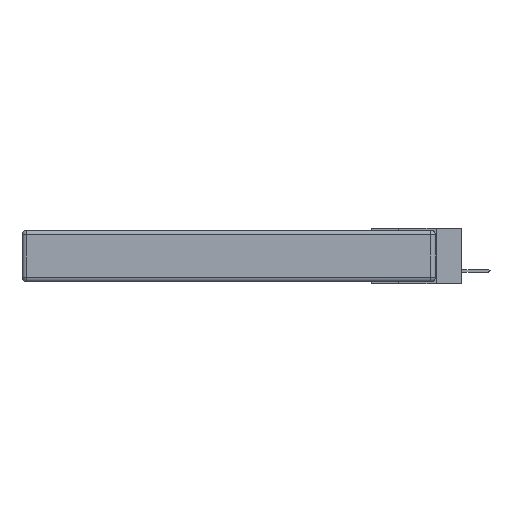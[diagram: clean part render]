
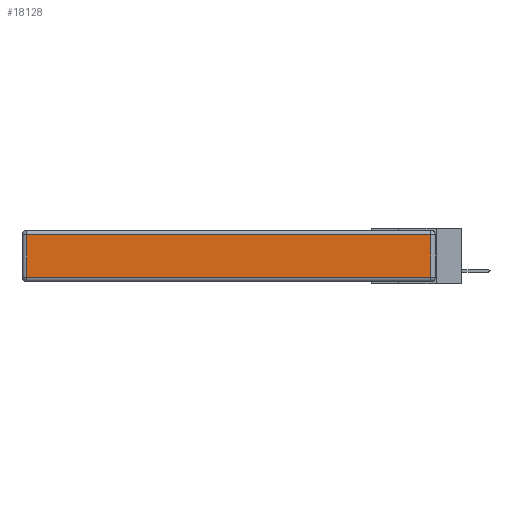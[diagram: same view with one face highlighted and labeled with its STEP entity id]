
A CAD part, left-side view. The second image highlights one B-rep face of the part: STEP entity #18128.
In plain terms, the highlighted planar face has unit normal (-1, 0, 0).
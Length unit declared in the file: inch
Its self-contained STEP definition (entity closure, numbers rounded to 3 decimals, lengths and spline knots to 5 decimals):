
#512 = VERTEX_POINT ( 'NONE', #15172 ) ;
#901 = VERTEX_POINT ( 'NONE', #2842 ) ;
#2226 = FACE_OUTER_BOUND ( 'NONE', #13156, .T. ) ;
#2771 = LINE ( 'NONE', #11736, #21294 ) ;
#2814 = ORIENTED_EDGE ( 'NONE', *, *, #7463, .T. ) ;
#2842 = CARTESIAN_POINT ( 'NONE',  ( 0., 0.03, -0.313 ) ) ;
#4754 = LINE ( 'NONE', #12436, #13782 ) ;
#5283 = DIRECTION ( 'NONE',  ( 0., 1., 0. ) ) ;
#5711 = DIRECTION ( 'NONE',  ( 0., 0., 1. ) ) ;
#6451 = DIRECTION ( 'NONE',  ( 0., 0., -1. ) ) ;
#6588 = ORIENTED_EDGE ( 'NONE', *, *, #10198, .T. ) ;
#7266 = ORIENTED_EDGE ( 'NONE', *, *, #14042, .T. ) ;
#7340 = LINE ( 'NONE', #15498, #22293 ) ;
#7463 = EDGE_CURVE ( 'NONE', #901, #9347, #4754, .T. ) ;
#8749 = ORIENTED_EDGE ( 'NONE', *, *, #14105, .T. ) ;
#9347 = VERTEX_POINT ( 'NONE', #15139 ) ;
#10198 = EDGE_CURVE ( 'NONE', #18504, #512, #2771, .T. ) ;
#10431 = DIRECTION ( 'NONE',  ( 0., 0., 1. ) ) ;
#11736 = CARTESIAN_POINT ( 'NONE',  ( 0., 2.72, -0.343 ) ) ;
#12436 = CARTESIAN_POINT ( 'NONE',  ( 0., 0.03, -0.343 ) ) ;
#13156 = EDGE_LOOP ( 'NONE', ( #7266, #2814, #8749, #6588 ) ) ;
#13782 = VECTOR ( 'NONE', #10431, 39.37008 ) ;
#14042 = EDGE_CURVE ( 'NONE', #512, #901, #16818, .T. ) ;
#14105 = EDGE_CURVE ( 'NONE', #9347, #18504, #7340, .T. ) ;
#15139 = CARTESIAN_POINT ( 'NONE',  ( 0., 0.03, -0.03 ) ) ;
#15172 = CARTESIAN_POINT ( 'NONE',  ( 0., 2.72, -0.313 ) ) ;
#15498 = CARTESIAN_POINT ( 'NONE',  ( 0., 2.75, -0.03 ) ) ;
#15646 = CARTESIAN_POINT ( 'NONE',  ( 0., 0., -0.313 ) ) ;
#15741 = CARTESIAN_POINT ( 'NONE',  ( 0., 2.72, -0.03 ) ) ;
#16292 = DIRECTION ( 'NONE',  ( -1., 0., 0. ) ) ;
#16294 = VECTOR ( 'NONE', #22416, 39.37008 ) ;
#16687 = AXIS2_PLACEMENT_3D ( 'NONE', #19951, #16292, #5711 ) ;
#16818 = LINE ( 'NONE', #15646, #16294 ) ;
#18126 = PLANE ( 'NONE',  #16687 ) ;
#18128 = ADVANCED_FACE ( 'NONE', ( #2226 ), #18126, .T. ) ;
#18504 = VERTEX_POINT ( 'NONE', #15741 ) ;
#19951 = CARTESIAN_POINT ( 'NONE',  ( 0., 0., -0.343 ) ) ;
#21294 = VECTOR ( 'NONE', #6451, 39.37008 ) ;
#22293 = VECTOR ( 'NONE', #5283, 39.37008 ) ;
#22416 = DIRECTION ( 'NONE',  ( 0., -1., 0. ) ) ;
